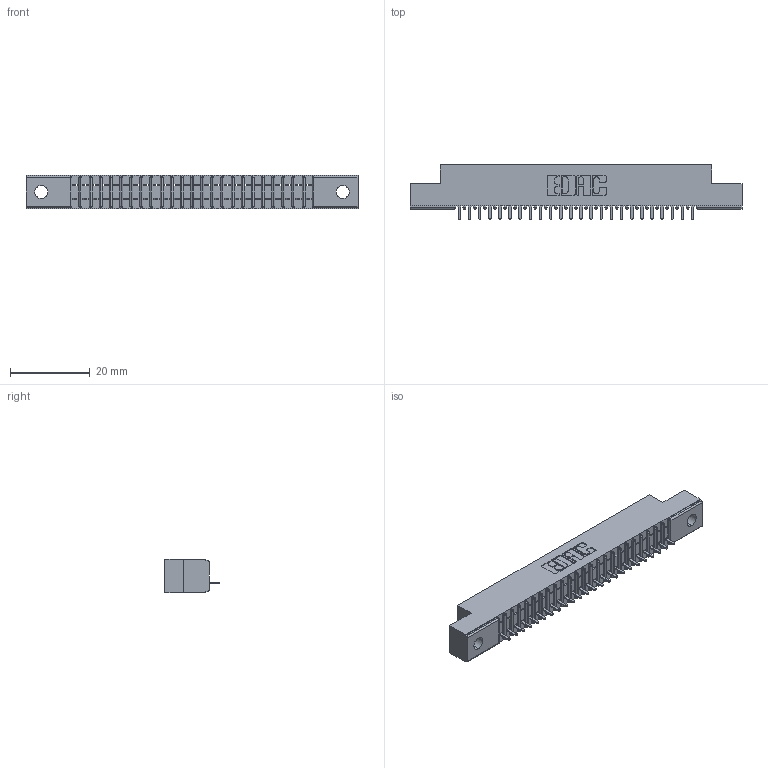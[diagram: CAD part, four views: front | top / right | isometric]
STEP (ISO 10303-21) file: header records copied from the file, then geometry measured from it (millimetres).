
FILE_DESCRIPTION (( 'STEP AP203' ), '1' );
FILE_NAME ('391-024-524-102.STEP', '2018-08-08T19:53:18', ( '' ), ( '' ), 'SwSTEP 2.0', 'SolidWorks 2016', '' );
FILE_SCHEMA (( 'CONFIG_CONTROL_DESIGN' ));
Length unit declared in the file: inch
Products named in the file (3): 341 Part_.128 (3.25) Dia Mounting Holes; 341-292-001_341-292-124; 391-024-524-102
Assembly tree (25 placements, depth 2):
  391-024-524-102
    341 Part_.128 (3.25) Dia Mounting Holes
    341-292-001_341-292-124  x24
Bounding box: 83.19 x 13.64 x 8.38 mm (x, y, z)
Volume: 4516.2 mm3; surface area: 8103 mm2
Topology: 25 solids, 25 shells, 2084 faces, 6004 edges, 3854 vertices
Faces by surface type: plane 1292, cylinder 696, sphere 50, torus 46
Entity records: 30677 total; most frequent: CARTESIAN_POINT 5204, ORIENTED_EDGE 5192, DIRECTION 5038, EDGE_CURVE 2596, VECTOR 2078, LINE 2078, VERTEX_POINT 1646, AXIS2_PLACEMENT_3D 1480
